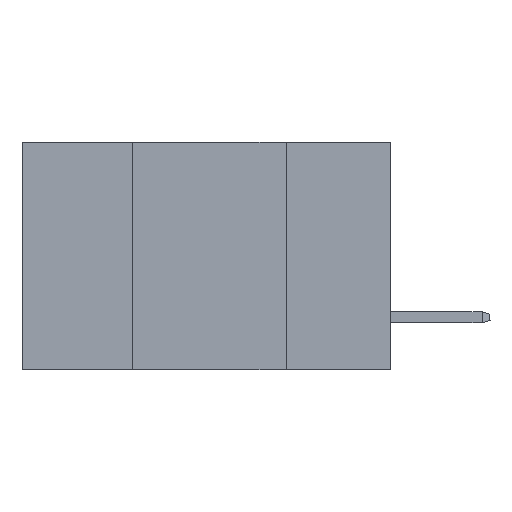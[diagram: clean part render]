
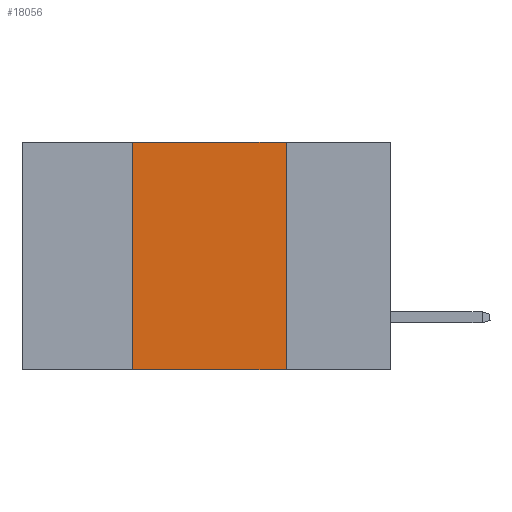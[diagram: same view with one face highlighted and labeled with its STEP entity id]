
A CAD part, left-side view. The second image highlights one B-rep face of the part: STEP entity #18056.
In plain terms, the highlighted planar face has unit normal (-1, 0, 0).
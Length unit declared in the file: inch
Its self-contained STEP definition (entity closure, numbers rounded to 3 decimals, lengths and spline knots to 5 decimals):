
#2 = ORIENTED_EDGE ( 'NONE', *, *, #24622, .F. ) ;
#888 = DIRECTION ( 'NONE',  ( 0., 0., -1. ) ) ;
#2137 = VECTOR ( 'NONE', #888, 39.37008 ) ;
#4031 = CARTESIAN_POINT ( 'NONE',  ( 0., 0.6, 0. ) ) ;
#5980 = VERTEX_POINT ( 'NONE', #19254 ) ;
#6257 = LINE ( 'NONE', #25228, #2137 ) ;
#6562 = FACE_OUTER_BOUND ( 'NONE', #18276, .T. ) ;
#6894 = AXIS2_PLACEMENT_3D ( 'NONE', #21054, #19019, #8775 ) ;
#7979 = LINE ( 'NONE', #4031, #14604 ) ;
#8298 = VECTOR ( 'NONE', #23955, 39.37008 ) ;
#8775 = DIRECTION ( 'NONE',  ( 0., 0., -1. ) ) ;
#10315 = EDGE_CURVE ( 'NONE', #18699, #12790, #23816, .T. ) ;
#10336 = CARTESIAN_POINT ( 'NONE',  ( 0., 0.17, -0.37 ) ) ;
#10440 = EDGE_CURVE ( 'NONE', #5980, #11955, #7979, .T. ) ;
#11058 = ORIENTED_EDGE ( 'NONE', *, *, #10315, .T. ) ;
#11955 = VERTEX_POINT ( 'NONE', #15566 ) ;
#12790 = VERTEX_POINT ( 'NONE', #10336 ) ;
#14604 = VECTOR ( 'NONE', #24446, 39.37008 ) ;
#14616 = PLANE ( 'NONE',  #6894 ) ;
#15566 = CARTESIAN_POINT ( 'NONE',  ( 0., 0.17, 0. ) ) ;
#17077 = DIRECTION ( 'NONE',  ( 0., 0., 1. ) ) ;
#18056 = ADVANCED_FACE ( 'NONE', ( #6562 ), #14616, .F. ) ;
#18127 = EDGE_CURVE ( 'NONE', #11955, #12790, #6257, .T. ) ;
#18276 = EDGE_LOOP ( 'NONE', ( #23887, #23547, #2, #11058 ) ) ;
#18394 = CARTESIAN_POINT ( 'NONE',  ( 0., 0.42, -0.37 ) ) ;
#18699 = VERTEX_POINT ( 'NONE', #18394 ) ;
#19019 = DIRECTION ( 'NONE',  ( 1., 0., 0. ) ) ;
#19254 = CARTESIAN_POINT ( 'NONE',  ( 0., 0.42, 0. ) ) ;
#19763 = VECTOR ( 'NONE', #17077, 39.37008 ) ;
#20995 = CARTESIAN_POINT ( 'NONE',  ( 0., 0.42, 0. ) ) ;
#21054 = CARTESIAN_POINT ( 'NONE',  ( 0., 0.6, 0. ) ) ;
#21790 = CARTESIAN_POINT ( 'NONE',  ( 0., 0.6, -0.37 ) ) ;
#23547 = ORIENTED_EDGE ( 'NONE', *, *, #10440, .F. ) ;
#23816 = LINE ( 'NONE', #21790, #8298 ) ;
#23887 = ORIENTED_EDGE ( 'NONE', *, *, #18127, .F. ) ;
#23955 = DIRECTION ( 'NONE',  ( 0., -1., 0. ) ) ;
#24446 = DIRECTION ( 'NONE',  ( 0., -1., 0. ) ) ;
#24510 = LINE ( 'NONE', #20995, #19763 ) ;
#24622 = EDGE_CURVE ( 'NONE', #18699, #5980, #24510, .T. ) ;
#25228 = CARTESIAN_POINT ( 'NONE',  ( 0., 0.17, 0. ) ) ;
